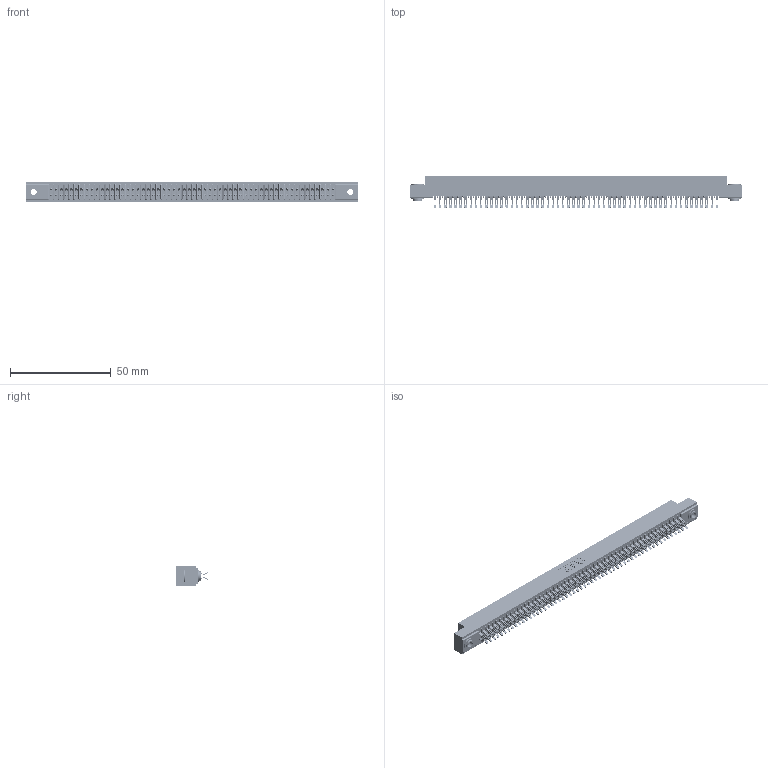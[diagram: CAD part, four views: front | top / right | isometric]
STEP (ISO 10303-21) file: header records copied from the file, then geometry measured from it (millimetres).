
FILE_DESCRIPTION (( 'STEP AP203' ), '1' );
FILE_NAME ('391-112-555-203.STEP', '2018-08-09T22:18:55', ( '' ), ( '' ), 'SwSTEP 2.0', 'SolidWorks 2016', '' );
FILE_SCHEMA (( 'CONFIG_CONTROL_DESIGN' ));
Length unit declared in the file: inch
Products named in the file (4): 345-250-002_345-250-002-102; 391-112-555-203; 341 Part_.156 (3.96) Dia Mounting Holes; 341-292-001_341-292-155
Assembly tree (115 placements, depth 2):
  391-112-555-203
    341 Part_.156 (3.96) Dia Mounting Holes
    341-292-001_341-292-155  x112
    345-250-002_345-250-002-102  x2
Bounding box: 164.47 x 16.31 x 10.16 mm (x, y, z)
Volume: 12300.9 mm3; surface area: 23436 mm2
Topology: 115 solids, 115 shells, 8904 faces, 26580 edges, 17302 vertices
Faces by surface type: plane 4796, cylinder 3876, sphere 114, torus 110, cone 8
Entity records: 67442 total; most frequent: CARTESIAN_POINT 11207, ORIENTED_EDGE 11120, DIRECTION 10872, EDGE_CURVE 5560, VECTOR 4482, LINE 4482, VERTEX_POINT 3514, AXIS2_PLACEMENT_3D 3195
